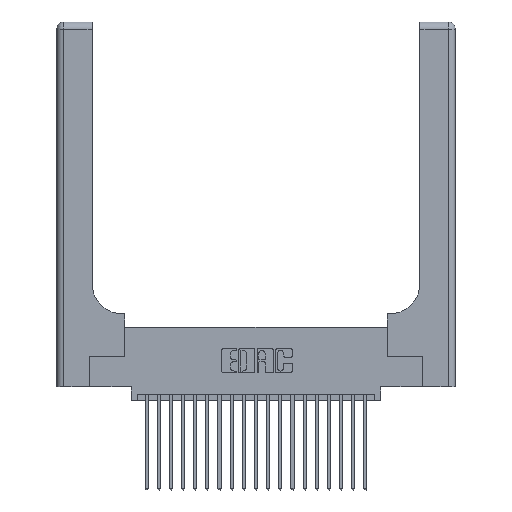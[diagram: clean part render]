
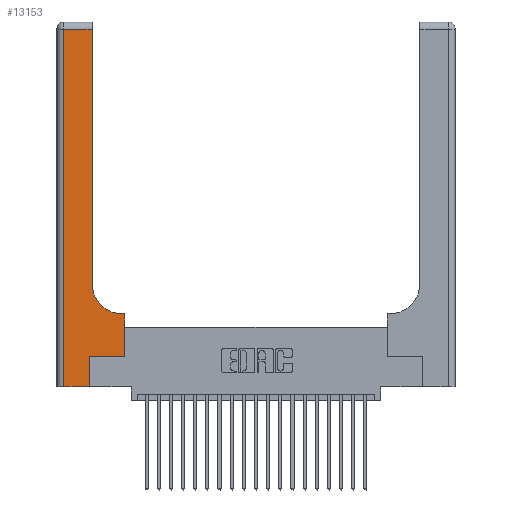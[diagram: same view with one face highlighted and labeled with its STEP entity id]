
A CAD part, top view. The second image highlights one B-rep face of the part: STEP entity #13153.
In plain terms, the highlighted planar face has unit normal (0, 0, 1).
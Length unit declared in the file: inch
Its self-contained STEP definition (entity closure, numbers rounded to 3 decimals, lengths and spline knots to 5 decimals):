
#583 = ORIENTED_EDGE ( 'NONE', *, *, #9633, .T. ) ;
#697 = EDGE_CURVE ( 'NONE', #17428, #17191, #18176, .T. ) ;
#1032 = ORIENTED_EDGE ( 'NONE', *, *, #9664, .T. ) ;
#1856 = DIRECTION ( 'NONE',  ( -1., 0., 0. ) ) ;
#2527 = EDGE_CURVE ( 'NONE', #5676, #13392, #21230, .T. ) ;
#2786 = CARTESIAN_POINT ( 'NONE',  ( 0.2915, 2.94, 0.37 ) ) ;
#2859 = DIRECTION ( 'NONE',  ( 0., 0., -1. ) ) ;
#3423 = LINE ( 'NONE', #23314, #17327 ) ;
#3495 = CARTESIAN_POINT ( 'NONE',  ( 0.06, 3., 0.37 ) ) ;
#3515 = CARTESIAN_POINT ( 'NONE',  ( 0.269, 0., 0.37 ) ) ;
#3762 = VECTOR ( 'NONE', #7286, 39.37008 ) ;
#4868 = VERTEX_POINT ( 'NONE', #15817 ) ;
#5118 = CARTESIAN_POINT ( 'NONE',  ( 0.2915, 0.85, 0.37 ) ) ;
#5351 = CARTESIAN_POINT ( 'NONE',  ( 0.5585, 0.25, 0.37 ) ) ;
#5375 = CARTESIAN_POINT ( 'NONE',  ( 0.2915, 0.6, 0.37 ) ) ;
#5486 = CARTESIAN_POINT ( 'NONE',  ( 0.2915, 3., 0.37 ) ) ;
#5676 = VERTEX_POINT ( 'NONE', #18317 ) ;
#6150 = CIRCLE ( 'NONE', #6404, 0.25 ) ;
#6305 = AXIS2_PLACEMENT_3D ( 'NONE', #10168, #2859, #15625 ) ;
#6404 = AXIS2_PLACEMENT_3D ( 'NONE', #18068, #7344, #19773 ) ;
#7221 = DIRECTION ( 'NONE',  ( -1., 0., 0. ) ) ;
#7242 = CARTESIAN_POINT ( 'NONE',  ( 0.269, 0.25, 0.37 ) ) ;
#7286 = DIRECTION ( 'NONE',  ( 1., 0., 0. ) ) ;
#7338 = DIRECTION ( 'NONE',  ( 0., 1., 0. ) ) ;
#7344 = DIRECTION ( 'NONE',  ( 0., 0., -1. ) ) ;
#7419 = DIRECTION ( 'NONE',  ( 0., 1., 0. ) ) ;
#7438 = EDGE_LOOP ( 'NONE', ( #10577, #7617, #14754, #14922, #583, #19865, #12804, #1032, #22381 ) ) ;
#7617 = ORIENTED_EDGE ( 'NONE', *, *, #12078, .T. ) ;
#8171 = VERTEX_POINT ( 'NONE', #2786 ) ;
#8705 = VERTEX_POINT ( 'NONE', #18899 ) ;
#9059 = EDGE_CURVE ( 'NONE', #17191, #22868, #16095, .T. ) ;
#9428 = DIRECTION ( 'NONE',  ( 1., 0., 0. ) ) ;
#9452 = FACE_OUTER_BOUND ( 'NONE', #7438, .T. ) ;
#9583 = LINE ( 'NONE', #5375, #17983 ) ;
#9633 = EDGE_CURVE ( 'NONE', #13392, #17428, #19581, .T. ) ;
#9664 = EDGE_CURVE ( 'NONE', #22868, #4868, #9583, .T. ) ;
#10168 = CARTESIAN_POINT ( 'NONE',  ( 0., 3., 0.37 ) ) ;
#10283 = EDGE_CURVE ( 'NONE', #4868, #11333, #6150, .T. ) ;
#10577 = ORIENTED_EDGE ( 'NONE', *, *, #18634, .T. ) ;
#11314 = VECTOR ( 'NONE', #7419, 39.37008 ) ;
#11333 = VERTEX_POINT ( 'NONE', #5118 ) ;
#11695 = CARTESIAN_POINT ( 'NONE',  ( 0.269, 0.25, 0.37 ) ) ;
#12078 = EDGE_CURVE ( 'NONE', #8171, #8705, #3423, .T. ) ;
#12540 = CARTESIAN_POINT ( 'NONE',  ( 0.269, 0., 0.37 ) ) ;
#12592 = EDGE_CURVE ( 'NONE', #8705, #5676, #17856, .T. ) ;
#12804 = ORIENTED_EDGE ( 'NONE', *, *, #9059, .T. ) ;
#13023 = LINE ( 'NONE', #5486, #21723 ) ;
#13153 = ADVANCED_FACE ( 'NONE', ( #9452 ), #13830, .F. ) ;
#13392 = VERTEX_POINT ( 'NONE', #3515 ) ;
#13830 = PLANE ( 'NONE',  #6305 ) ;
#14331 = DIRECTION ( 'NONE',  ( 0., 1., 0. ) ) ;
#14396 = VECTOR ( 'NONE', #14331, 39.37008 ) ;
#14754 = ORIENTED_EDGE ( 'NONE', *, *, #12592, .T. ) ;
#14922 = ORIENTED_EDGE ( 'NONE', *, *, #2527, .T. ) ;
#15625 = DIRECTION ( 'NONE',  ( -1., 0., 0. ) ) ;
#15817 = CARTESIAN_POINT ( 'NONE',  ( 0.5415, 0.6, 0.37 ) ) ;
#16095 = LINE ( 'NONE', #21475, #11314 ) ;
#17191 = VERTEX_POINT ( 'NONE', #5351 ) ;
#17327 = VECTOR ( 'NONE', #1856, 39.37008 ) ;
#17428 = VERTEX_POINT ( 'NONE', #11695 ) ;
#17856 = LINE ( 'NONE', #3495, #18396 ) ;
#17973 = DIRECTION ( 'NONE',  ( 0., -1., 0. ) ) ;
#17983 = VECTOR ( 'NONE', #7221, 39.37008 ) ;
#18068 = CARTESIAN_POINT ( 'NONE',  ( 0.5415, 0.85, 0.37 ) ) ;
#18176 = LINE ( 'NONE', #7242, #3762 ) ;
#18317 = CARTESIAN_POINT ( 'NONE',  ( 0.06, 0., 0.37 ) ) ;
#18396 = VECTOR ( 'NONE', #17973, 39.37008 ) ;
#18634 = EDGE_CURVE ( 'NONE', #11333, #8171, #13023, .T. ) ;
#18899 = CARTESIAN_POINT ( 'NONE',  ( 0.06, 2.94, 0.37 ) ) ;
#19581 = LINE ( 'NONE', #12540, #14396 ) ;
#19773 = DIRECTION ( 'NONE',  ( 1., 0., 0. ) ) ;
#19865 = ORIENTED_EDGE ( 'NONE', *, *, #697, .T. ) ;
#20046 = CARTESIAN_POINT ( 'NONE',  ( 0., 0., 0.37 ) ) ;
#21230 = LINE ( 'NONE', #20046, #21768 ) ;
#21429 = CARTESIAN_POINT ( 'NONE',  ( 0.5585, 0.6, 0.37 ) ) ;
#21475 = CARTESIAN_POINT ( 'NONE',  ( 0.5585, 0.25, 0.37 ) ) ;
#21723 = VECTOR ( 'NONE', #7338, 39.37008 ) ;
#21768 = VECTOR ( 'NONE', #9428, 39.37008 ) ;
#22381 = ORIENTED_EDGE ( 'NONE', *, *, #10283, .T. ) ;
#22868 = VERTEX_POINT ( 'NONE', #21429 ) ;
#23314 = CARTESIAN_POINT ( 'NONE',  ( 0., 2.94, 0.37 ) ) ;
